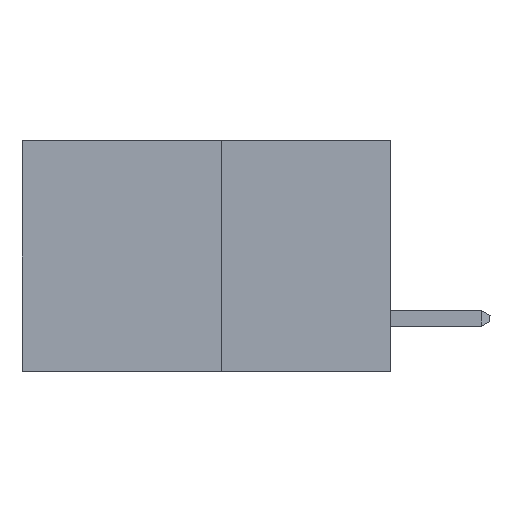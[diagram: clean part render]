
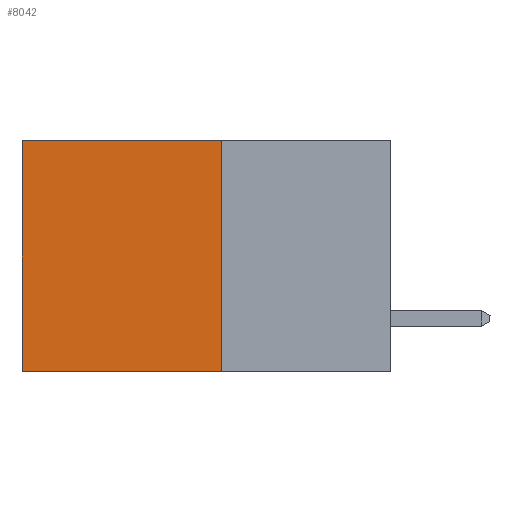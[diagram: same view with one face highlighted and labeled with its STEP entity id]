
A CAD part, left-side view. The second image highlights one B-rep face of the part: STEP entity #8042.
In plain terms, the highlighted planar face has unit normal (-1, 0, 0).
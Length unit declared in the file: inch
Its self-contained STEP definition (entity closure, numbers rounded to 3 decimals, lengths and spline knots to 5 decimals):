
#224 = DIRECTION ( 'NONE',  ( 0., 1., 0. ) ) ;
#1362 = VERTEX_POINT ( 'NONE', #7544 ) ;
#1553 = LINE ( 'NONE', #2459, #6719 ) ;
#1998 = EDGE_CURVE ( 'NONE', #1362, #13092, #5236, .T. ) ;
#2168 = CARTESIAN_POINT ( 'NONE',  ( 0.277, 0.59, 0. ) ) ;
#2459 = CARTESIAN_POINT ( 'NONE',  ( 0.277, 0.27, 0. ) ) ;
#3154 = EDGE_LOOP ( 'NONE', ( #10161, #7729, #12260, #10637 ) ) ;
#3918 = EDGE_CURVE ( 'NONE', #5200, #6804, #7971, .T. ) ;
#4082 = CARTESIAN_POINT ( 'NONE',  ( 0.277, 0.27, -0.37 ) ) ;
#4721 = EDGE_CURVE ( 'NONE', #1362, #5200, #1553, .T. ) ;
#4763 = EDGE_CURVE ( 'NONE', #13092, #6804, #6064, .T. ) ;
#5130 = DIRECTION ( 'NONE',  ( 1., 0., 0. ) ) ;
#5200 = VERTEX_POINT ( 'NONE', #2168 ) ;
#5236 = LINE ( 'NONE', #8756, #7703 ) ;
#6064 = LINE ( 'NONE', #7898, #11110 ) ;
#6719 = VECTOR ( 'NONE', #11765, 39.37008 ) ;
#6804 = VERTEX_POINT ( 'NONE', #10686 ) ;
#7544 = CARTESIAN_POINT ( 'NONE',  ( 0.277, 0.27, 0. ) ) ;
#7653 = VECTOR ( 'NONE', #9989, 39.37008 ) ;
#7703 = VECTOR ( 'NONE', #8393, 39.37008 ) ;
#7729 = ORIENTED_EDGE ( 'NONE', *, *, #4763, .F. ) ;
#7898 = CARTESIAN_POINT ( 'NONE',  ( 0.277, 0.27, -0.37 ) ) ;
#7971 = LINE ( 'NONE', #10152, #7653 ) ;
#8042 = ADVANCED_FACE ( 'NONE', ( #11508 ), #10219, .F. ) ;
#8393 = DIRECTION ( 'NONE',  ( 0., 0., -1. ) ) ;
#8756 = CARTESIAN_POINT ( 'NONE',  ( 0.277, 0.27, -0.37 ) ) ;
#8790 = AXIS2_PLACEMENT_3D ( 'NONE', #4082, #5130, #12213 ) ;
#9989 = DIRECTION ( 'NONE',  ( 0., 0., -1. ) ) ;
#10152 = CARTESIAN_POINT ( 'NONE',  ( 0.277, 0.59, -0.37 ) ) ;
#10161 = ORIENTED_EDGE ( 'NONE', *, *, #3918, .T. ) ;
#10219 = PLANE ( 'NONE',  #8790 ) ;
#10593 = CARTESIAN_POINT ( 'NONE',  ( 0.277, 0.27, -0.37 ) ) ;
#10637 = ORIENTED_EDGE ( 'NONE', *, *, #4721, .T. ) ;
#10686 = CARTESIAN_POINT ( 'NONE',  ( 0.277, 0.59, -0.37 ) ) ;
#11110 = VECTOR ( 'NONE', #224, 39.37008 ) ;
#11508 = FACE_OUTER_BOUND ( 'NONE', #3154, .T. ) ;
#11765 = DIRECTION ( 'NONE',  ( 0., 1., 0. ) ) ;
#12213 = DIRECTION ( 'NONE',  ( 0., 0., -1. ) ) ;
#12260 = ORIENTED_EDGE ( 'NONE', *, *, #1998, .F. ) ;
#13092 = VERTEX_POINT ( 'NONE', #10593 ) ;
